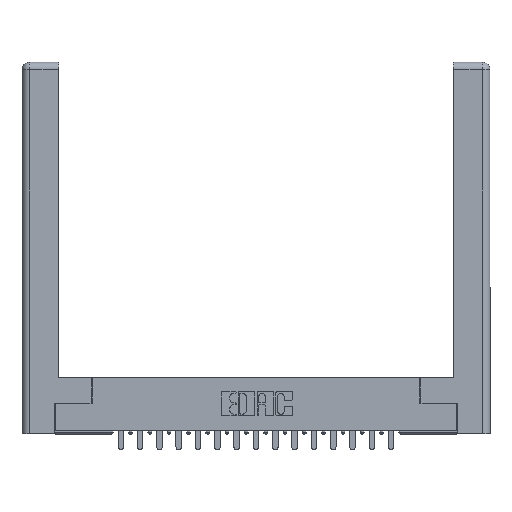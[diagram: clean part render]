
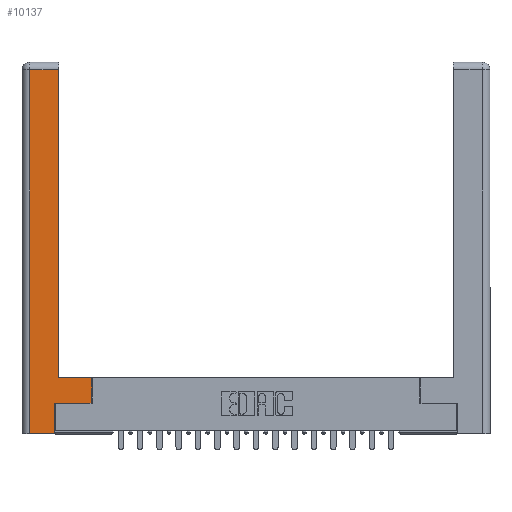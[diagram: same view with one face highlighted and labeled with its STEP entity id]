
A CAD part, top view. The second image highlights one B-rep face of the part: STEP entity #10137.
In plain terms, the highlighted planar face has unit normal (0, 0, 1).
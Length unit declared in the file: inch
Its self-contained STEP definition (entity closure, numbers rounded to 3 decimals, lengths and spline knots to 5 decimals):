
#867 = LINE ( 'NONE', #18317, #19800 ) ;
#1162 = LINE ( 'NONE', #16917, #12350 ) ;
#1215 = CARTESIAN_POINT ( 'NONE',  ( 0.295, 0.45, 0. ) ) ;
#1693 = DIRECTION ( 'NONE',  ( 1., 0., 0. ) ) ;
#1973 = CARTESIAN_POINT ( 'NONE',  ( 0.565, 0.245, 0. ) ) ;
#2221 = ORIENTED_EDGE ( 'NONE', *, *, #16622, .T. ) ;
#2384 = VERTEX_POINT ( 'NONE', #21090 ) ;
#2585 = DIRECTION ( 'NONE',  ( -1., 0., 0. ) ) ;
#2746 = CARTESIAN_POINT ( 'NONE',  ( 0.265, 0., 0. ) ) ;
#3082 = ORIENTED_EDGE ( 'NONE', *, *, #20063, .T. ) ;
#3454 = CARTESIAN_POINT ( 'NONE',  ( 0.0615, 2.94, 0. ) ) ;
#3894 = CARTESIAN_POINT ( 'NONE',  ( 0., 0., 0. ) ) ;
#4037 = DIRECTION ( 'NONE',  ( 0., -1., 0. ) ) ;
#4091 = EDGE_CURVE ( 'NONE', #2384, #7117, #1162, .T. ) ;
#4268 = LINE ( 'NONE', #1215, #19737 ) ;
#4608 = VECTOR ( 'NONE', #4037, 39.37008 ) ;
#4742 = VERTEX_POINT ( 'NONE', #2746 ) ;
#4981 = EDGE_CURVE ( 'NONE', #4742, #2384, #867, .T. ) ;
#5217 = ORIENTED_EDGE ( 'NONE', *, *, #12435, .T. ) ;
#5797 = VERTEX_POINT ( 'NONE', #8923 ) ;
#5946 = VECTOR ( 'NONE', #1693, 39.37008 ) ;
#6352 = VERTEX_POINT ( 'NONE', #17030 ) ;
#6656 = VERTEX_POINT ( 'NONE', #11262 ) ;
#6900 = CARTESIAN_POINT ( 'NONE',  ( 0.0615, 2.94, 0. ) ) ;
#6906 = VECTOR ( 'NONE', #8229, 39.37008 ) ;
#7117 = VERTEX_POINT ( 'NONE', #1973 ) ;
#7491 = AXIS2_PLACEMENT_3D ( 'NONE', #3894, #7741, #2585 ) ;
#7741 = DIRECTION ( 'NONE',  ( 0., 0., -1. ) ) ;
#7882 = DIRECTION ( 'NONE',  ( -1., 0., 0. ) ) ;
#8229 = DIRECTION ( 'NONE',  ( 0., 1., 0. ) ) ;
#8276 = VERTEX_POINT ( 'NONE', #3454 ) ;
#8356 = VECTOR ( 'NONE', #13814, 39.37008 ) ;
#8372 = EDGE_CURVE ( 'NONE', #6656, #6352, #21215, .T. ) ;
#8382 = DIRECTION ( 'NONE',  ( 1., 0., 0. ) ) ;
#8923 = CARTESIAN_POINT ( 'NONE',  ( 0.565, 0.45, 0. ) ) ;
#8977 = EDGE_LOOP ( 'NONE', ( #20115, #12256, #3082, #2221, #13290, #15805, #19260, #5217 ) ) ;
#9990 = DIRECTION ( 'NONE',  ( 0., 1., 0. ) ) ;
#10137 = ADVANCED_FACE ( 'NONE', ( #15277 ), #14245, .F. ) ;
#10487 = LINE ( 'NONE', #11358, #5946 ) ;
#11117 = EDGE_CURVE ( 'NONE', #7117, #5797, #16549, .T. ) ;
#11262 = CARTESIAN_POINT ( 'NONE',  ( 0.295, 0.45, 0. ) ) ;
#11350 = DIRECTION ( 'NONE',  ( 0., 1., 0. ) ) ;
#11358 = CARTESIAN_POINT ( 'NONE',  ( 0.265, 0., 0. ) ) ;
#12256 = ORIENTED_EDGE ( 'NONE', *, *, #16386, .T. ) ;
#12350 = VECTOR ( 'NONE', #8382, 39.37008 ) ;
#12435 = EDGE_CURVE ( 'NONE', #5797, #6656, #4268, .T. ) ;
#12918 = LINE ( 'NONE', #6900, #8356 ) ;
#13290 = ORIENTED_EDGE ( 'NONE', *, *, #4981, .T. ) ;
#13462 = CARTESIAN_POINT ( 'NONE',  ( 0.565, 0.45, 0. ) ) ;
#13518 = CARTESIAN_POINT ( 'NONE',  ( 0.0615, 0., 0. ) ) ;
#13814 = DIRECTION ( 'NONE',  ( -1., 0., 0. ) ) ;
#14245 = PLANE ( 'NONE',  #7491 ) ;
#15277 = FACE_OUTER_BOUND ( 'NONE', #8977, .T. ) ;
#15380 = CARTESIAN_POINT ( 'NONE',  ( 0.295, 3., 0. ) ) ;
#15805 = ORIENTED_EDGE ( 'NONE', *, *, #4091, .T. ) ;
#16082 = LINE ( 'NONE', #16275, #4608 ) ;
#16275 = CARTESIAN_POINT ( 'NONE',  ( 0.0615, 0., 0. ) ) ;
#16386 = EDGE_CURVE ( 'NONE', #6352, #8276, #12918, .T. ) ;
#16549 = LINE ( 'NONE', #13462, #6906 ) ;
#16622 = EDGE_CURVE ( 'NONE', #21660, #4742, #10487, .T. ) ;
#16917 = CARTESIAN_POINT ( 'NONE',  ( 0.565, 0.245, 0. ) ) ;
#17030 = CARTESIAN_POINT ( 'NONE',  ( 0.295, 2.94, 0. ) ) ;
#18317 = CARTESIAN_POINT ( 'NONE',  ( 0.265, 0.245, 0. ) ) ;
#18855 = VECTOR ( 'NONE', #9990, 39.37008 ) ;
#19260 = ORIENTED_EDGE ( 'NONE', *, *, #11117, .T. ) ;
#19737 = VECTOR ( 'NONE', #7882, 39.37008 ) ;
#19800 = VECTOR ( 'NONE', #11350, 39.37008 ) ;
#20063 = EDGE_CURVE ( 'NONE', #8276, #21660, #16082, .T. ) ;
#20115 = ORIENTED_EDGE ( 'NONE', *, *, #8372, .T. ) ;
#21090 = CARTESIAN_POINT ( 'NONE',  ( 0.265, 0.245, 0. ) ) ;
#21215 = LINE ( 'NONE', #15380, #18855 ) ;
#21660 = VERTEX_POINT ( 'NONE', #13518 ) ;
